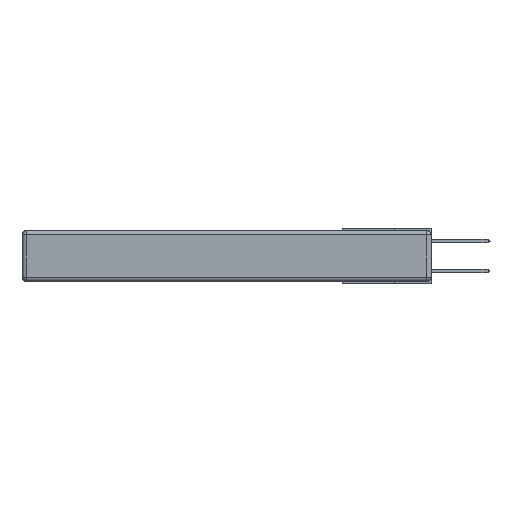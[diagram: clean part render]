
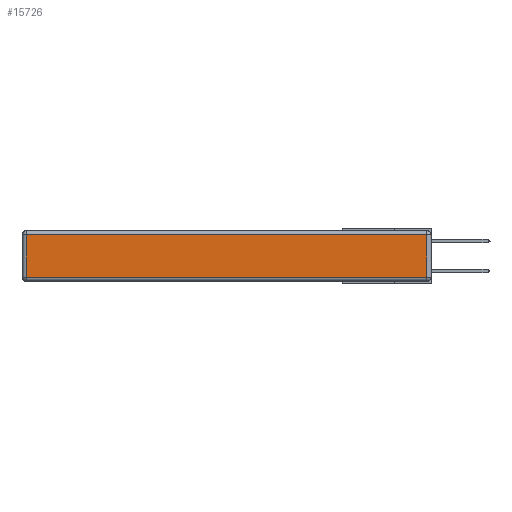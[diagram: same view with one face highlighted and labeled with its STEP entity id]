
A CAD part, left-side view. The second image highlights one B-rep face of the part: STEP entity #15726.
In plain terms, the highlighted planar face has unit normal (-1, 0, 0).
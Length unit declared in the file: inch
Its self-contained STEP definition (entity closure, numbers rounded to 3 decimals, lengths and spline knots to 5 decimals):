
#181 = DIRECTION ( 'NONE',  ( 0., 0., -1. ) ) ;
#1231 = VERTEX_POINT ( 'NONE', #14832 ) ;
#2921 = DIRECTION ( 'NONE',  ( 0., 0., 1. ) ) ;
#3749 = EDGE_CURVE ( 'NONE', #14200, #1231, #22215, .T. ) ;
#3985 = DIRECTION ( 'NONE',  ( 0., -1., 0. ) ) ;
#4489 = ORIENTED_EDGE ( 'NONE', *, *, #19396, .T. ) ;
#4774 = DIRECTION ( 'NONE',  ( 0., 0., 1. ) ) ;
#6538 = PLANE ( 'NONE',  #20071 ) ;
#6761 = CARTESIAN_POINT ( 'NONE',  ( 0., 2.72, -0.313 ) ) ;
#8192 = DIRECTION ( 'NONE',  ( 0., 1., 0. ) ) ;
#8582 = VECTOR ( 'NONE', #4774, 39.37008 ) ;
#9004 = CARTESIAN_POINT ( 'NONE',  ( 0., 0.03, -0.03 ) ) ;
#9551 = EDGE_CURVE ( 'NONE', #1231, #13923, #20972, .T. ) ;
#9584 = ORIENTED_EDGE ( 'NONE', *, *, #10059, .T. ) ;
#9630 = EDGE_LOOP ( 'NONE', ( #21834, #19273, #9584, #4489 ) ) ;
#10059 = EDGE_CURVE ( 'NONE', #13923, #14477, #20951, .T. ) ;
#10859 = VECTOR ( 'NONE', #181, 39.37008 ) ;
#11334 = VECTOR ( 'NONE', #3985, 39.37008 ) ;
#13427 = CARTESIAN_POINT ( 'NONE',  ( 0., 0., -0.313 ) ) ;
#13923 = VERTEX_POINT ( 'NONE', #9004 ) ;
#14200 = VERTEX_POINT ( 'NONE', #6761 ) ;
#14477 = VERTEX_POINT ( 'NONE', #23633 ) ;
#14832 = CARTESIAN_POINT ( 'NONE',  ( 0., 0.03, -0.313 ) ) ;
#15726 = ADVANCED_FACE ( 'NONE', ( #17424 ), #6538, .T. ) ;
#17424 = FACE_OUTER_BOUND ( 'NONE', #9630, .T. ) ;
#17820 = CARTESIAN_POINT ( 'NONE',  ( 0., 2.75, -0.03 ) ) ;
#18360 = CARTESIAN_POINT ( 'NONE',  ( 0., 0.03, -0.343 ) ) ;
#19273 = ORIENTED_EDGE ( 'NONE', *, *, #9551, .T. ) ;
#19396 = EDGE_CURVE ( 'NONE', #14477, #14200, #21163, .T. ) ;
#20071 = AXIS2_PLACEMENT_3D ( 'NONE', #20398, #22244, #2921 ) ;
#20398 = CARTESIAN_POINT ( 'NONE',  ( 0., 0., -0.343 ) ) ;
#20951 = LINE ( 'NONE', #17820, #21554 ) ;
#20972 = LINE ( 'NONE', #18360, #8582 ) ;
#21163 = LINE ( 'NONE', #23229, #10859 ) ;
#21554 = VECTOR ( 'NONE', #8192, 39.37008 ) ;
#21834 = ORIENTED_EDGE ( 'NONE', *, *, #3749, .T. ) ;
#22215 = LINE ( 'NONE', #13427, #11334 ) ;
#22244 = DIRECTION ( 'NONE',  ( -1., 0., 0. ) ) ;
#23229 = CARTESIAN_POINT ( 'NONE',  ( 0., 2.72, -0.343 ) ) ;
#23633 = CARTESIAN_POINT ( 'NONE',  ( 0., 2.72, -0.03 ) ) ;
